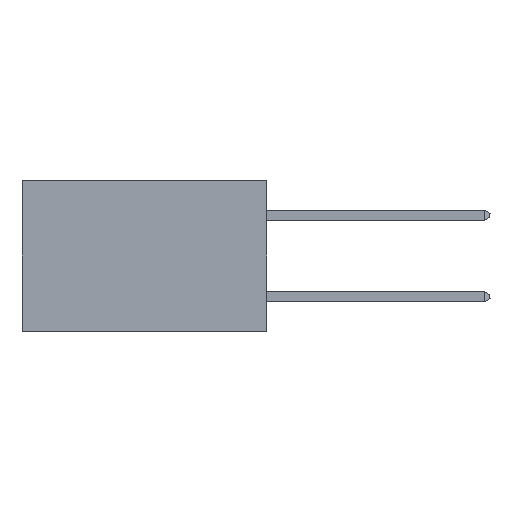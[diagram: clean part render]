
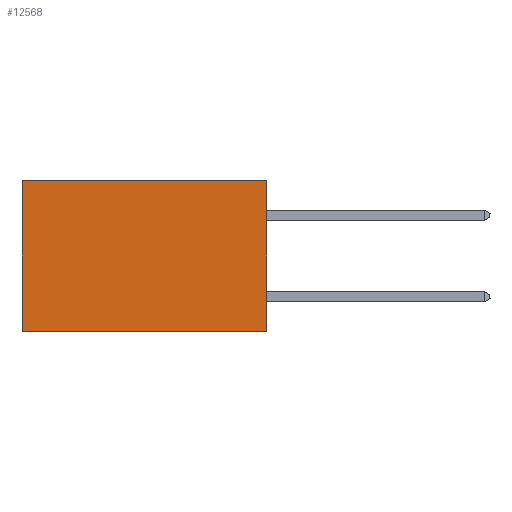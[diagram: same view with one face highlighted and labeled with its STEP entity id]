
A CAD part, left-side view. The second image highlights one B-rep face of the part: STEP entity #12568.
In plain terms, the highlighted planar face has unit normal (-1, 0, 0).
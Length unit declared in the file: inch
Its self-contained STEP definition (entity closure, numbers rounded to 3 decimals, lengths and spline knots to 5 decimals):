
#675 = LINE ( 'NONE', #10330, #12158 ) ;
#1324 = DIRECTION ( 'NONE',  ( 0., 1., 0. ) ) ;
#1464 = EDGE_CURVE ( 'NONE', #7805, #9905, #675, .T. ) ;
#1601 = VERTEX_POINT ( 'NONE', #2836 ) ;
#1835 = VERTEX_POINT ( 'NONE', #3162 ) ;
#2435 = LINE ( 'NONE', #5805, #18116 ) ;
#2640 = DIRECTION ( 'NONE',  ( 1., 0., 0. ) ) ;
#2836 = CARTESIAN_POINT ( 'NONE',  ( 0.2875, 0., 0. ) ) ;
#3162 = CARTESIAN_POINT ( 'NONE',  ( 0.2875, 0., -0.37 ) ) ;
#4285 = AXIS2_PLACEMENT_3D ( 'NONE', #7439, #2640, #19235 ) ;
#5399 = DIRECTION ( 'NONE',  ( 0., 0., -1. ) ) ;
#5805 = CARTESIAN_POINT ( 'NONE',  ( 0.2875, 0., 0. ) ) ;
#6163 = ORIENTED_EDGE ( 'NONE', *, *, #1464, .T. ) ;
#6591 = CARTESIAN_POINT ( 'NONE',  ( 0.2875, 0.6, -0.37 ) ) ;
#7439 = CARTESIAN_POINT ( 'NONE',  ( 0.2875, 0., 0. ) ) ;
#7805 = VERTEX_POINT ( 'NONE', #18113 ) ;
#7939 = EDGE_CURVE ( 'NONE', #1835, #9905, #16984, .T. ) ;
#8349 = LINE ( 'NONE', #14940, #16728 ) ;
#9827 = EDGE_LOOP ( 'NONE', ( #6163, #18981, #18575, #11863 ) ) ;
#9905 = VERTEX_POINT ( 'NONE', #6591 ) ;
#10330 = CARTESIAN_POINT ( 'NONE',  ( 0.2875, 0.6, 0. ) ) ;
#11863 = ORIENTED_EDGE ( 'NONE', *, *, #18983, .T. ) ;
#11900 = EDGE_CURVE ( 'NONE', #1601, #1835, #2435, .T. ) ;
#12158 = VECTOR ( 'NONE', #5399, 39.37008 ) ;
#12568 = ADVANCED_FACE ( 'NONE', ( #13059 ), #17621, .F. ) ;
#13059 = FACE_OUTER_BOUND ( 'NONE', #9827, .T. ) ;
#14940 = CARTESIAN_POINT ( 'NONE',  ( 0.2875, 0., 0. ) ) ;
#16651 = DIRECTION ( 'NONE',  ( 0., 1., 0. ) ) ;
#16728 = VECTOR ( 'NONE', #16651, 39.37008 ) ;
#16984 = LINE ( 'NONE', #17998, #19616 ) ;
#17621 = PLANE ( 'NONE',  #4285 ) ;
#17998 = CARTESIAN_POINT ( 'NONE',  ( 0.2875, 0., -0.37 ) ) ;
#18113 = CARTESIAN_POINT ( 'NONE',  ( 0.2875, 0.6, 0. ) ) ;
#18116 = VECTOR ( 'NONE', #20885, 39.37008 ) ;
#18575 = ORIENTED_EDGE ( 'NONE', *, *, #11900, .F. ) ;
#18981 = ORIENTED_EDGE ( 'NONE', *, *, #7939, .F. ) ;
#18983 = EDGE_CURVE ( 'NONE', #1601, #7805, #8349, .T. ) ;
#19235 = DIRECTION ( 'NONE',  ( 0., 0., -1. ) ) ;
#19616 = VECTOR ( 'NONE', #1324, 39.37008 ) ;
#20885 = DIRECTION ( 'NONE',  ( 0., 0., -1. ) ) ;
